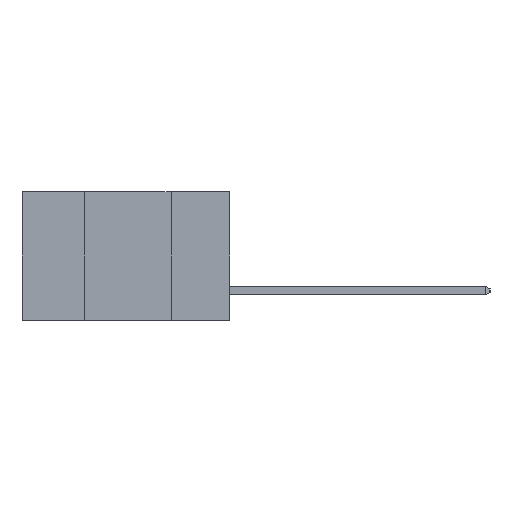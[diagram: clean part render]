
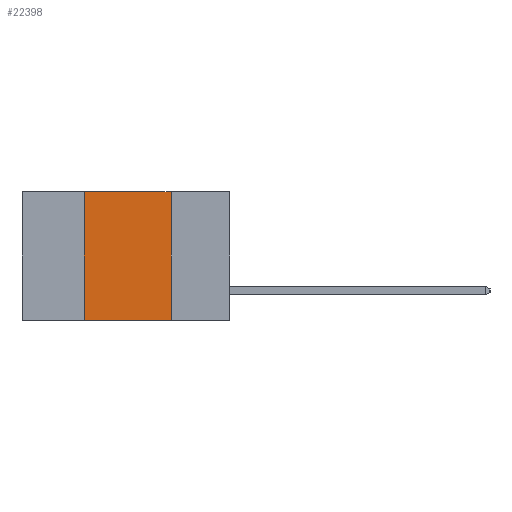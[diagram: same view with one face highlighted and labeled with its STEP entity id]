
A CAD part, left-side view. The second image highlights one B-rep face of the part: STEP entity #22398.
In plain terms, the highlighted planar face has unit normal (-1, 0, 0).
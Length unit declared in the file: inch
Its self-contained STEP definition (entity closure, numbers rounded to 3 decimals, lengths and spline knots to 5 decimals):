
#501 = VERTEX_POINT ( 'NONE', #8097 ) ;
#1083 = VECTOR ( 'NONE', #4277, 39.37008 ) ;
#1165 = EDGE_CURVE ( 'NONE', #10708, #7877, #14600, .T. ) ;
#1736 = LINE ( 'NONE', #14210, #1083 ) ;
#1899 = PLANE ( 'NONE',  #14270 ) ;
#3089 = CARTESIAN_POINT ( 'NONE',  ( 0., 0.42, 0. ) ) ;
#3880 = CARTESIAN_POINT ( 'NONE',  ( 0., 0.6, -0.37 ) ) ;
#3937 = DIRECTION ( 'NONE',  ( 0., 0., -1. ) ) ;
#4277 = DIRECTION ( 'NONE',  ( 0., 0., -1. ) ) ;
#7395 = CARTESIAN_POINT ( 'NONE',  ( 0., 0.17, 0. ) ) ;
#7697 = ORIENTED_EDGE ( 'NONE', *, *, #22322, .F. ) ;
#7765 = CARTESIAN_POINT ( 'NONE',  ( 0., 0.6, 0. ) ) ;
#7877 = VERTEX_POINT ( 'NONE', #7395 ) ;
#7926 = CARTESIAN_POINT ( 'NONE',  ( 0., 0.6, 0. ) ) ;
#8041 = DIRECTION ( 'NONE',  ( 0., -1., 0. ) ) ;
#8097 = CARTESIAN_POINT ( 'NONE',  ( 0., 0.17, -0.37 ) ) ;
#8193 = EDGE_CURVE ( 'NONE', #7877, #501, #1736, .T. ) ;
#9339 = VECTOR ( 'NONE', #14886, 39.37008 ) ;
#9742 = CARTESIAN_POINT ( 'NONE',  ( 0., 0.42, 0. ) ) ;
#10708 = VERTEX_POINT ( 'NONE', #3089 ) ;
#11725 = ORIENTED_EDGE ( 'NONE', *, *, #8193, .F. ) ;
#11730 = DIRECTION ( 'NONE',  ( 0., 0., 1. ) ) ;
#12129 = LINE ( 'NONE', #3880, #21458 ) ;
#12139 = VECTOR ( 'NONE', #11730, 39.37008 ) ;
#14210 = CARTESIAN_POINT ( 'NONE',  ( 0., 0.17, 0. ) ) ;
#14270 = AXIS2_PLACEMENT_3D ( 'NONE', #7926, #15901, #3937 ) ;
#14600 = LINE ( 'NONE', #7765, #9339 ) ;
#14656 = VERTEX_POINT ( 'NONE', #19325 ) ;
#14886 = DIRECTION ( 'NONE',  ( 0., -1., 0. ) ) ;
#15901 = DIRECTION ( 'NONE',  ( 1., 0., 0. ) ) ;
#16481 = EDGE_LOOP ( 'NONE', ( #11725, #17660, #7697, #18907 ) ) ;
#17442 = LINE ( 'NONE', #9742, #12139 ) ;
#17660 = ORIENTED_EDGE ( 'NONE', *, *, #1165, .F. ) ;
#18907 = ORIENTED_EDGE ( 'NONE', *, *, #24435, .T. ) ;
#19325 = CARTESIAN_POINT ( 'NONE',  ( 0., 0.42, -0.37 ) ) ;
#20851 = FACE_OUTER_BOUND ( 'NONE', #16481, .T. ) ;
#21458 = VECTOR ( 'NONE', #8041, 39.37008 ) ;
#22322 = EDGE_CURVE ( 'NONE', #14656, #10708, #17442, .T. ) ;
#22398 = ADVANCED_FACE ( 'NONE', ( #20851 ), #1899, .F. ) ;
#24435 = EDGE_CURVE ( 'NONE', #14656, #501, #12129, .T. ) ;
